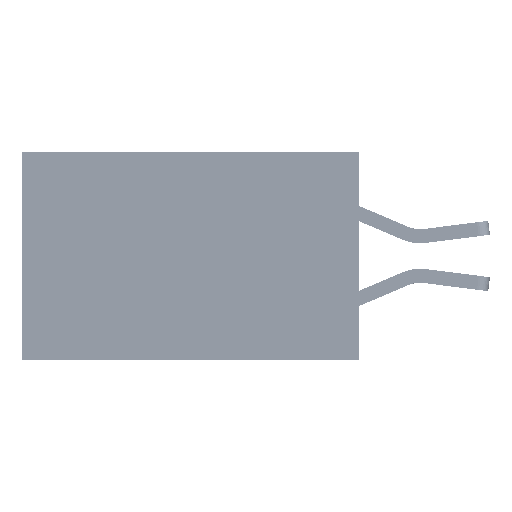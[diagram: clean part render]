
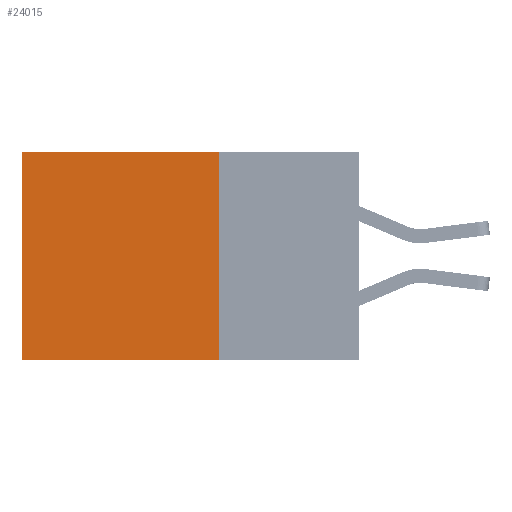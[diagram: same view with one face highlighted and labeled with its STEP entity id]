
A CAD part, left-side view. The second image highlights one B-rep face of the part: STEP entity #24015.
In plain terms, the highlighted planar face has unit normal (-1, 0, 0).
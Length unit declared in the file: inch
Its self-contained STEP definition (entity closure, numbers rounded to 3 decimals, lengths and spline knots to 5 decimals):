
#68 = VERTEX_POINT ( 'NONE', #30879 ) ;
#138 = AXIS2_PLACEMENT_3D ( 'NONE', #14563, #35271, #15023 ) ;
#589 = CARTESIAN_POINT ( 'NONE',  ( 0.2875, 0.25, 0. ) ) ;
#1432 = EDGE_CURVE ( 'NONE', #68, #32550, #34118, .T. ) ;
#2269 = ORIENTED_EDGE ( 'NONE', *, *, #32778, .F. ) ;
#6085 = CARTESIAN_POINT ( 'NONE',  ( 0.2875, 0.6, 0. ) ) ;
#6552 = ORIENTED_EDGE ( 'NONE', *, *, #26637, .F. ) ;
#8953 = CARTESIAN_POINT ( 'NONE',  ( 0.2875, 0.25, -0.37 ) ) ;
#9579 = CARTESIAN_POINT ( 'NONE',  ( 0.2875, 0.25, 0. ) ) ;
#11704 = DIRECTION ( 'NONE',  ( 0., 1., 0. ) ) ;
#14563 = CARTESIAN_POINT ( 'NONE',  ( 0.2875, 0.25, 0. ) ) ;
#15023 = DIRECTION ( 'NONE',  ( 0., 0., -1. ) ) ;
#16429 = DIRECTION ( 'NONE',  ( 0., 0., -1. ) ) ;
#18141 = VERTEX_POINT ( 'NONE', #18423 ) ;
#18423 = CARTESIAN_POINT ( 'NONE',  ( 0.2875, 0.25, -0.37 ) ) ;
#20481 = ORIENTED_EDGE ( 'NONE', *, *, #1432, .T. ) ;
#23503 = EDGE_CURVE ( 'NONE', #38046, #68, #27044, .T. ) ;
#23819 = DIRECTION ( 'NONE',  ( 0., 1., 0. ) ) ;
#24015 = ADVANCED_FACE ( 'NONE', ( #32265 ), #28595, .F. ) ;
#24852 = VECTOR ( 'NONE', #11704, 39.37008 ) ;
#25517 = EDGE_LOOP ( 'NONE', ( #20481, #2269, #6552, #29639 ) ) ;
#26329 = CARTESIAN_POINT ( 'NONE',  ( 0.2875, 0.6, -0.37 ) ) ;
#26520 = VECTOR ( 'NONE', #16429, 39.37008 ) ;
#26637 = EDGE_CURVE ( 'NONE', #38046, #18141, #38782, .T. ) ;
#27044 = LINE ( 'NONE', #9579, #30941 ) ;
#28224 = DIRECTION ( 'NONE',  ( 0., 0., -1. ) ) ;
#28595 = PLANE ( 'NONE',  #138 ) ;
#28700 = VECTOR ( 'NONE', #28224, 39.37008 ) ;
#29639 = ORIENTED_EDGE ( 'NONE', *, *, #23503, .T. ) ;
#30879 = CARTESIAN_POINT ( 'NONE',  ( 0.2875, 0.6, 0. ) ) ;
#30941 = VECTOR ( 'NONE', #23819, 39.37008 ) ;
#32265 = FACE_OUTER_BOUND ( 'NONE', #25517, .T. ) ;
#32550 = VERTEX_POINT ( 'NONE', #26329 ) ;
#32778 = EDGE_CURVE ( 'NONE', #18141, #32550, #40444, .T. ) ;
#34118 = LINE ( 'NONE', #6085, #26520 ) ;
#35271 = DIRECTION ( 'NONE',  ( 1., 0., 0. ) ) ;
#38046 = VERTEX_POINT ( 'NONE', #589 ) ;
#38782 = LINE ( 'NONE', #39030, #28700 ) ;
#39030 = CARTESIAN_POINT ( 'NONE',  ( 0.2875, 0.25, 0. ) ) ;
#40444 = LINE ( 'NONE', #8953, #24852 ) ;
